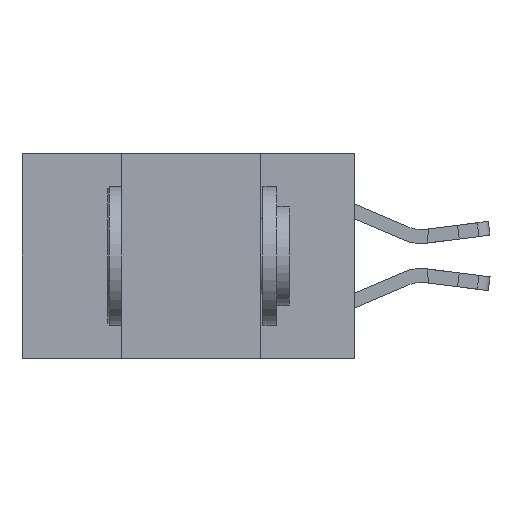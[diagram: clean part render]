
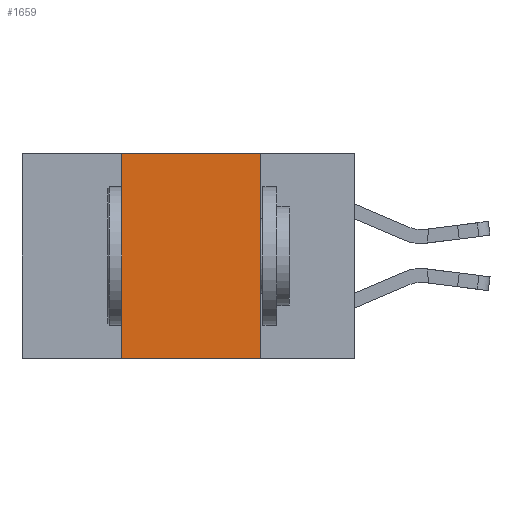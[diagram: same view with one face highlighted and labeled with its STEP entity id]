
A CAD part, left-side view. The second image highlights one B-rep face of the part: STEP entity #1659.
In plain terms, the highlighted planar face has unit normal (-1, 0, 0).
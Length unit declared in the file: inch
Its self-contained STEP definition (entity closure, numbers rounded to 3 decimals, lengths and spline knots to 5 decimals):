
#271 = ORIENTED_EDGE ( 'NONE', *, *, #3033, .F. ) ;
#704 = FACE_OUTER_BOUND ( 'NONE', #1548, .T. ) ;
#803 = CARTESIAN_POINT ( 'NONE',  ( 0., 0.6, -0.37 ) ) ;
#900 = CARTESIAN_POINT ( 'NONE',  ( 0., 0.6, 0. ) ) ;
#1266 = VECTOR ( 'NONE', #14136, 39.37008 ) ;
#1548 = EDGE_LOOP ( 'NONE', ( #1662, #271, #12536, #12017 ) ) ;
#1578 = CARTESIAN_POINT ( 'NONE',  ( 0., 0.42, -0.37 ) ) ;
#1659 = ADVANCED_FACE ( 'NONE', ( #704 ), #5314, .F. ) ;
#1662 = ORIENTED_EDGE ( 'NONE', *, *, #12303, .F. ) ;
#1749 = DIRECTION ( 'NONE',  ( 0., -1., 0. ) ) ;
#2346 = VECTOR ( 'NONE', #9998, 39.37008 ) ;
#3033 = EDGE_CURVE ( 'NONE', #6777, #4244, #5391, .T. ) ;
#3299 = CARTESIAN_POINT ( 'NONE',  ( 0., 0.17, 0. ) ) ;
#3339 = LINE ( 'NONE', #4795, #10636 ) ;
#4125 = DIRECTION ( 'NONE',  ( 0., 0., -1. ) ) ;
#4244 = VERTEX_POINT ( 'NONE', #3299 ) ;
#4521 = CARTESIAN_POINT ( 'NONE',  ( 0., 0.17, 0. ) ) ;
#4795 = CARTESIAN_POINT ( 'NONE',  ( 0., 0.42, 0. ) ) ;
#5314 = PLANE ( 'NONE',  #6109 ) ;
#5343 = LINE ( 'NONE', #4521, #2346 ) ;
#5391 = LINE ( 'NONE', #13826, #14141 ) ;
#5678 = EDGE_CURVE ( 'NONE', #8455, #8839, #10788, .T. ) ;
#5873 = DIRECTION ( 'NONE',  ( 0., 0., 1. ) ) ;
#6109 = AXIS2_PLACEMENT_3D ( 'NONE', #900, #12929, #4125 ) ;
#6777 = VERTEX_POINT ( 'NONE', #10239 ) ;
#8272 = EDGE_CURVE ( 'NONE', #8455, #6777, #3339, .T. ) ;
#8455 = VERTEX_POINT ( 'NONE', #1578 ) ;
#8839 = VERTEX_POINT ( 'NONE', #13803 ) ;
#9998 = DIRECTION ( 'NONE',  ( 0., 0., -1. ) ) ;
#10239 = CARTESIAN_POINT ( 'NONE',  ( 0., 0.42, 0. ) ) ;
#10636 = VECTOR ( 'NONE', #5873, 39.37008 ) ;
#10788 = LINE ( 'NONE', #803, #1266 ) ;
#12017 = ORIENTED_EDGE ( 'NONE', *, *, #5678, .T. ) ;
#12303 = EDGE_CURVE ( 'NONE', #4244, #8839, #5343, .T. ) ;
#12536 = ORIENTED_EDGE ( 'NONE', *, *, #8272, .F. ) ;
#12929 = DIRECTION ( 'NONE',  ( 1., 0., 0. ) ) ;
#13803 = CARTESIAN_POINT ( 'NONE',  ( 0., 0.17, -0.37 ) ) ;
#13826 = CARTESIAN_POINT ( 'NONE',  ( 0., 0.6, 0. ) ) ;
#14136 = DIRECTION ( 'NONE',  ( 0., -1., 0. ) ) ;
#14141 = VECTOR ( 'NONE', #1749, 39.37008 ) ;
